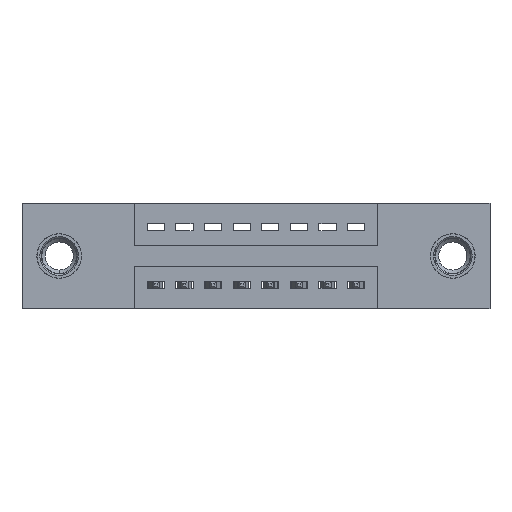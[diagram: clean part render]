
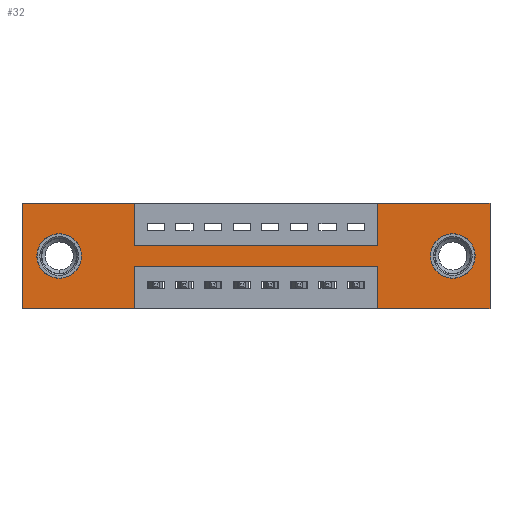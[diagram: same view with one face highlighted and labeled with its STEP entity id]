
A CAD part, front view. The second image highlights one B-rep face of the part: STEP entity #32.
In plain terms, the highlighted planar face has unit normal (0, -1, 0).
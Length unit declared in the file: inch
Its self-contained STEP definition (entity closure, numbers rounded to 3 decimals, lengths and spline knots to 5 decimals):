
#6 = CARTESIAN_POINT ( 'NONE',  ( 1.2425, 0., -0.37 ) ) ;
#32 = ADVANCED_FACE ( 'NONE', ( #6041, #7471, #8043 ), #9350, .T. ) ;
#189 = VERTEX_POINT ( 'NONE', #704 ) ;
#325 = CARTESIAN_POINT ( 'NONE',  ( 1.2425, 0., 0. ) ) ;
#590 = LINE ( 'NONE', #4974, #10716 ) ;
#642 = CARTESIAN_POINT ( 'NONE',  ( 0., 0., 0. ) ) ;
#704 = CARTESIAN_POINT ( 'NONE',  ( 0.3925, 0., 0. ) ) ;
#760 = LINE ( 'NONE', #6, #11181 ) ;
#807 = CIRCLE ( 'NONE', #11607, 0.078 ) ;
#825 = EDGE_CURVE ( 'NONE', #2902, #3718, #6292, .T. ) ;
#924 = EDGE_LOOP ( 'NONE', ( #5888, #5651, #5347, #11392, #6817, #11540, #1068, #10228, #6621, #11565, #10348, #11486 ) ) ;
#1068 = ORIENTED_EDGE ( 'NONE', *, *, #2901, .F. ) ;
#1101 = VECTOR ( 'NONE', #7035, 39.37008 ) ;
#1111 = EDGE_CURVE ( 'NONE', #6469, #10367, #2142, .T. ) ;
#1214 = CARTESIAN_POINT ( 'NONE',  ( 1.635, 0., 0. ) ) ;
#1248 = EDGE_CURVE ( 'NONE', #6943, #4190, #2275, .T. ) ;
#1277 = DIRECTION ( 'NONE',  ( 1., 0., 0. ) ) ;
#1349 = EDGE_LOOP ( 'NONE', ( #8894, #1464 ) ) ;
#1383 = AXIS2_PLACEMENT_3D ( 'NONE', #10286, #3999, #4881 ) ;
#1396 = CARTESIAN_POINT ( 'NONE',  ( 1.2425, 0., 0. ) ) ;
#1464 = ORIENTED_EDGE ( 'NONE', *, *, #9584, .T. ) ;
#1489 = VECTOR ( 'NONE', #6231, 39.37008 ) ;
#1566 = CARTESIAN_POINT ( 'NONE',  ( 0.3925, 0., 0. ) ) ;
#1580 = CARTESIAN_POINT ( 'NONE',  ( 1.2425, 0., -0.37 ) ) ;
#1678 = LINE ( 'NONE', #7438, #7128 ) ;
#1810 = LINE ( 'NONE', #325, #1101 ) ;
#1866 = DIRECTION ( 'NONE',  ( 0., 1., 0. ) ) ;
#1970 = CARTESIAN_POINT ( 'NONE',  ( 1.635, 0., -0.37 ) ) ;
#1999 = LINE ( 'NONE', #3997, #2296 ) ;
#2142 = LINE ( 'NONE', #4965, #11548 ) ;
#2238 = DIRECTION ( 'NONE',  ( -1., 0., 0. ) ) ;
#2271 = EDGE_CURVE ( 'NONE', #5304, #6469, #1678, .T. ) ;
#2275 = LINE ( 'NONE', #3457, #10985 ) ;
#2276 = CARTESIAN_POINT ( 'NONE',  ( 0.3925, 0., -0.22 ) ) ;
#2296 = VECTOR ( 'NONE', #1277, 39.37008 ) ;
#2491 = DIRECTION ( 'NONE',  ( 0., 1., 0. ) ) ;
#2540 = EDGE_CURVE ( 'NONE', #2638, #4706, #4690, .T. ) ;
#2638 = VERTEX_POINT ( 'NONE', #1970 ) ;
#2901 = EDGE_CURVE ( 'NONE', #4190, #3224, #1810, .T. ) ;
#2902 = VERTEX_POINT ( 'NONE', #11525 ) ;
#2928 = DIRECTION ( 'NONE',  ( 0., 0., -1. ) ) ;
#2956 = AXIS2_PLACEMENT_3D ( 'NONE', #3880, #6594, #5857 ) ;
#3074 = CARTESIAN_POINT ( 'NONE',  ( 0.3925, 0., -0.22 ) ) ;
#3136 = EDGE_CURVE ( 'NONE', #5715, #6945, #807, .T. ) ;
#3224 = VERTEX_POINT ( 'NONE', #1396 ) ;
#3271 = VECTOR ( 'NONE', #6234, 39.37008 ) ;
#3455 = EDGE_CURVE ( 'NONE', #9723, #189, #590, .T. ) ;
#3457 = CARTESIAN_POINT ( 'NONE',  ( 0.3925, 0., -0.15 ) ) ;
#3530 = CARTESIAN_POINT ( 'NONE',  ( 0., 0., -0.37 ) ) ;
#3620 = DIRECTION ( 'NONE',  ( 0., 0., -1. ) ) ;
#3718 = VERTEX_POINT ( 'NONE', #4417 ) ;
#3880 = CARTESIAN_POINT ( 'NONE',  ( 1.505, 0., -0.185 ) ) ;
#3971 = LINE ( 'NONE', #1566, #1489 ) ;
#3980 = CARTESIAN_POINT ( 'NONE',  ( 0.13, 0., -0.263 ) ) ;
#3997 = CARTESIAN_POINT ( 'NONE',  ( 0., 0., 0. ) ) ;
#3999 = DIRECTION ( 'NONE',  ( 0., 1., 0. ) ) ;
#4033 = CARTESIAN_POINT ( 'NONE',  ( 1.2425, 0., -0.15 ) ) ;
#4052 = DIRECTION ( 'NONE',  ( -1., 0., 0. ) ) ;
#4070 = CIRCLE ( 'NONE', #1383, 0.078 ) ;
#4086 = AXIS2_PLACEMENT_3D ( 'NONE', #9151, #8375, #3620 ) ;
#4175 = CARTESIAN_POINT ( 'NONE',  ( 0., 0., -0.37 ) ) ;
#4190 = VERTEX_POINT ( 'NONE', #4033 ) ;
#4197 = EDGE_CURVE ( 'NONE', #3224, #7120, #1999, .T. ) ;
#4221 = CARTESIAN_POINT ( 'NONE',  ( 0., 0., 0. ) ) ;
#4417 = CARTESIAN_POINT ( 'NONE',  ( 1.505, 0., -0.263 ) ) ;
#4463 = CARTESIAN_POINT ( 'NONE',  ( 0.13, 0., -0.107 ) ) ;
#4690 = LINE ( 'NONE', #3530, #3271 ) ;
#4706 = VERTEX_POINT ( 'NONE', #1580 ) ;
#4809 = LINE ( 'NONE', #3074, #8662 ) ;
#4881 = DIRECTION ( 'NONE',  ( 0., 0., 1. ) ) ;
#4962 = EDGE_CURVE ( 'NONE', #7120, #2638, #9854, .T. ) ;
#4965 = CARTESIAN_POINT ( 'NONE',  ( 0., 0., -0.37 ) ) ;
#4974 = CARTESIAN_POINT ( 'NONE',  ( 0., 0., 0. ) ) ;
#5013 = VECTOR ( 'NONE', #11278, 39.37008 ) ;
#5222 = VERTEX_POINT ( 'NONE', #8457 ) ;
#5304 = VERTEX_POINT ( 'NONE', #2276 ) ;
#5347 = ORIENTED_EDGE ( 'NONE', *, *, #8682, .F. ) ;
#5651 = ORIENTED_EDGE ( 'NONE', *, *, #10850, .F. ) ;
#5715 = VERTEX_POINT ( 'NONE', #4463 ) ;
#5857 = DIRECTION ( 'NONE',  ( 0., 0., -1. ) ) ;
#5888 = ORIENTED_EDGE ( 'NONE', *, *, #2271, .F. ) ;
#6041 = FACE_BOUND ( 'NONE', #6702, .T. ) ;
#6116 = ORIENTED_EDGE ( 'NONE', *, *, #7099, .T. ) ;
#6136 = CARTESIAN_POINT ( 'NONE',  ( 1.505, 0., -0.185 ) ) ;
#6231 = DIRECTION ( 'NONE',  ( 0., 0., -1. ) ) ;
#6234 = DIRECTION ( 'NONE',  ( -1., 0., 0. ) ) ;
#6292 = CIRCLE ( 'NONE', #6562, 0.078 ) ;
#6469 = VERTEX_POINT ( 'NONE', #9042 ) ;
#6562 = AXIS2_PLACEMENT_3D ( 'NONE', #6136, #2491, #9827 ) ;
#6594 = DIRECTION ( 'NONE',  ( 0., 1., 0. ) ) ;
#6621 = ORIENTED_EDGE ( 'NONE', *, *, #8285, .F. ) ;
#6702 = EDGE_LOOP ( 'NONE', ( #7001, #6116 ) ) ;
#6817 = ORIENTED_EDGE ( 'NONE', *, *, #4962, .F. ) ;
#6943 = VERTEX_POINT ( 'NONE', #7541 ) ;
#6945 = VERTEX_POINT ( 'NONE', #3980 ) ;
#7001 = ORIENTED_EDGE ( 'NONE', *, *, #825, .T. ) ;
#7031 = DIRECTION ( 'NONE',  ( 0., 0., 1. ) ) ;
#7035 = DIRECTION ( 'NONE',  ( 0., 0., 1. ) ) ;
#7099 = EDGE_CURVE ( 'NONE', #3718, #2902, #8401, .T. ) ;
#7120 = VERTEX_POINT ( 'NONE', #1214 ) ;
#7128 = VECTOR ( 'NONE', #2928, 39.37008 ) ;
#7298 = DIRECTION ( 'NONE',  ( 0., 0., 1. ) ) ;
#7326 = EDGE_CURVE ( 'NONE', #10367, #9723, #9089, .T. ) ;
#7438 = CARTESIAN_POINT ( 'NONE',  ( 0.3925, 0., -0.37 ) ) ;
#7471 = FACE_BOUND ( 'NONE', #1349, .T. ) ;
#7541 = CARTESIAN_POINT ( 'NONE',  ( 0.3925, 0., -0.15 ) ) ;
#7811 = VECTOR ( 'NONE', #7031, 39.37008 ) ;
#8043 = FACE_OUTER_BOUND ( 'NONE', #924, .T. ) ;
#8271 = DIRECTION ( 'NONE',  ( 1., 0., 0. ) ) ;
#8285 = EDGE_CURVE ( 'NONE', #189, #6943, #3971, .T. ) ;
#8375 = DIRECTION ( 'NONE',  ( 0., -1., 0. ) ) ;
#8401 = CIRCLE ( 'NONE', #2956, 0.078 ) ;
#8457 = CARTESIAN_POINT ( 'NONE',  ( 1.2425, 0., -0.22 ) ) ;
#8662 = VECTOR ( 'NONE', #4052, 39.37008 ) ;
#8682 = EDGE_CURVE ( 'NONE', #4706, #5222, #760, .T. ) ;
#8894 = ORIENTED_EDGE ( 'NONE', *, *, #3136, .T. ) ;
#9042 = CARTESIAN_POINT ( 'NONE',  ( 0.3925, 0., -0.37 ) ) ;
#9089 = LINE ( 'NONE', #642, #7811 ) ;
#9151 = CARTESIAN_POINT ( 'NONE',  ( 0., 0., -0.37 ) ) ;
#9350 = PLANE ( 'NONE',  #4086 ) ;
#9387 = CARTESIAN_POINT ( 'NONE',  ( 1.635, 0., 0. ) ) ;
#9520 = DIRECTION ( 'NONE',  ( 1., 0., 0. ) ) ;
#9584 = EDGE_CURVE ( 'NONE', #6945, #5715, #4070, .T. ) ;
#9723 = VERTEX_POINT ( 'NONE', #4221 ) ;
#9827 = DIRECTION ( 'NONE',  ( 0., 0., -1. ) ) ;
#9854 = LINE ( 'NONE', #9387, #5013 ) ;
#10228 = ORIENTED_EDGE ( 'NONE', *, *, #1248, .F. ) ;
#10286 = CARTESIAN_POINT ( 'NONE',  ( 0.13, 0., -0.185 ) ) ;
#10348 = ORIENTED_EDGE ( 'NONE', *, *, #7326, .F. ) ;
#10367 = VERTEX_POINT ( 'NONE', #4175 ) ;
#10716 = VECTOR ( 'NONE', #9520, 39.37008 ) ;
#10850 = EDGE_CURVE ( 'NONE', #5222, #5304, #4809, .T. ) ;
#10931 = CARTESIAN_POINT ( 'NONE',  ( 0.13, 0., -0.185 ) ) ;
#10985 = VECTOR ( 'NONE', #8271, 39.37008 ) ;
#11175 = DIRECTION ( 'NONE',  ( 0., 0., 1. ) ) ;
#11181 = VECTOR ( 'NONE', #7298, 39.37008 ) ;
#11278 = DIRECTION ( 'NONE',  ( 0., 0., -1. ) ) ;
#11392 = ORIENTED_EDGE ( 'NONE', *, *, #2540, .F. ) ;
#11486 = ORIENTED_EDGE ( 'NONE', *, *, #1111, .F. ) ;
#11525 = CARTESIAN_POINT ( 'NONE',  ( 1.505, 0., -0.107 ) ) ;
#11540 = ORIENTED_EDGE ( 'NONE', *, *, #4197, .F. ) ;
#11548 = VECTOR ( 'NONE', #2238, 39.37008 ) ;
#11565 = ORIENTED_EDGE ( 'NONE', *, *, #3455, .F. ) ;
#11607 = AXIS2_PLACEMENT_3D ( 'NONE', #10931, #1866, #11175 ) ;
